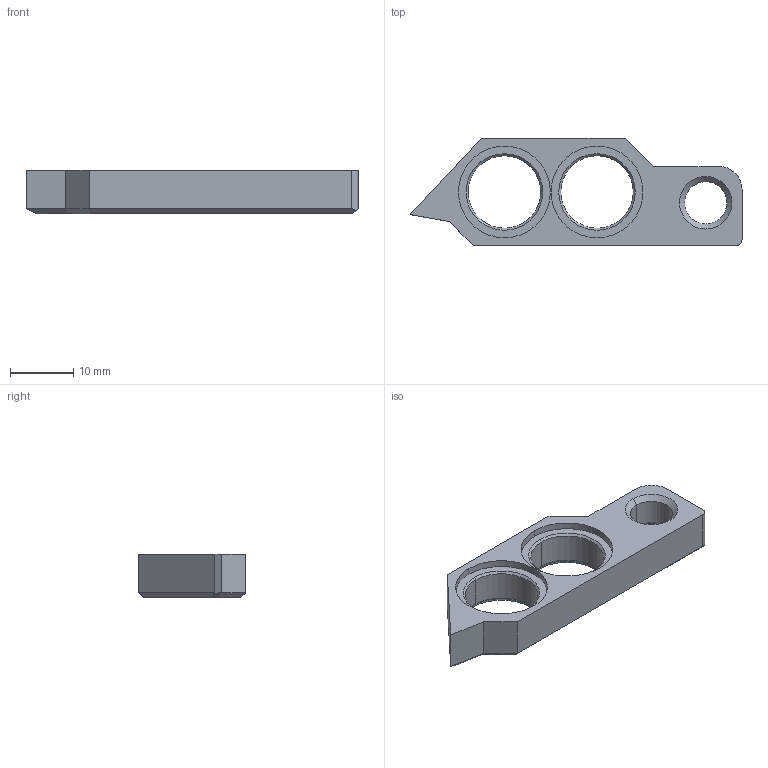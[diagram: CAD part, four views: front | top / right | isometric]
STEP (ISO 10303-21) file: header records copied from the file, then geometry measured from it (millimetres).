
FILE_DESCRIPTION (( 'STEP AP203' ), '1' );
FILE_NAME ('AF-HF-LR-PRT-005-STEP.STEP', '2020-11-05T07:10:09', ( '' ), ( '' ), 'SwSTEP 2.0', 'SolidWorks 2018', '' );
FILE_SCHEMA (( 'CONFIG_CONTROL_DESIGN' ));
Length unit declared in the file: inch
Products named in the file (1): AF-HF-LR-PRT-005-STEP
Bounding box: 52.35 x 16.89 x 6.91 mm (x, y, z)
Volume: 3008.2 mm3; surface area: 2353.6 mm2
Topology: 1 solids, 1 shells, 51 faces, 115 edges, 68 vertices
Faces by surface type: plane 20, cylinder 18, cone 13
Entity records: 1494 total; most frequent: DIRECTION 259, CARTESIAN_POINT 241, ORIENTED_EDGE 230, EDGE_CURVE 115, AXIS2_PLACEMENT_3D 94, VECTOR 71, LINE 71, VERTEX_POINT 68
